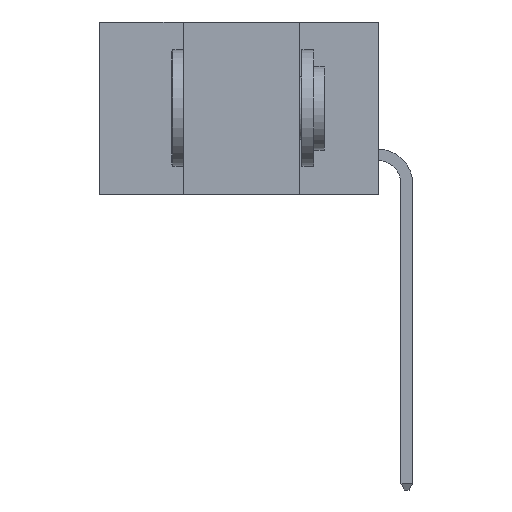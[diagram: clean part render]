
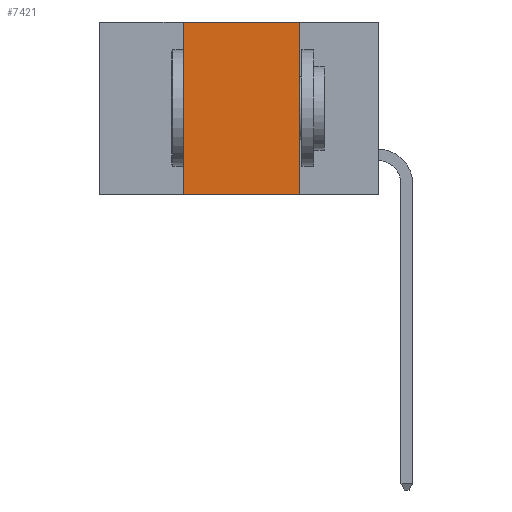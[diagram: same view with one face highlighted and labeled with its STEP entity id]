
A CAD part, left-side view. The second image highlights one B-rep face of the part: STEP entity #7421.
In plain terms, the highlighted planar face has unit normal (-1, 0, 0).
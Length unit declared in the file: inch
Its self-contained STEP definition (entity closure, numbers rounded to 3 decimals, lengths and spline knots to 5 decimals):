
#63 = LINE ( 'NONE', #23181, #14083 ) ;
#337 = CARTESIAN_POINT ( 'NONE',  ( 0., 0.17, -0.37 ) ) ;
#1043 = EDGE_CURVE ( 'NONE', #14700, #1186, #8381, .T. ) ;
#1186 = VERTEX_POINT ( 'NONE', #1383 ) ;
#1383 = CARTESIAN_POINT ( 'NONE',  ( 0., 0.17, -0.37 ) ) ;
#1869 = VECTOR ( 'NONE', #4277, 39.37008 ) ;
#3516 = EDGE_CURVE ( 'NONE', #14700, #6450, #6801, .T. ) ;
#4277 = DIRECTION ( 'NONE',  ( 0., 0., 1. ) ) ;
#4461 = DIRECTION ( 'NONE',  ( 0., 0., -1. ) ) ;
#6450 = VERTEX_POINT ( 'NONE', #11587 ) ;
#6664 = AXIS2_PLACEMENT_3D ( 'NONE', #16986, #16760, #16734 ) ;
#6705 = CARTESIAN_POINT ( 'NONE',  ( 0., 0.6, -0.37 ) ) ;
#6801 = LINE ( 'NONE', #8044, #1869 ) ;
#7071 = FACE_OUTER_BOUND ( 'NONE', #11452, .T. ) ;
#7185 = CARTESIAN_POINT ( 'NONE',  ( 0., 0.17, 0. ) ) ;
#7223 = VECTOR ( 'NONE', #11606, 39.37008 ) ;
#7421 = ADVANCED_FACE ( 'NONE', ( #7071 ), #16840, .F. ) ;
#8044 = CARTESIAN_POINT ( 'NONE',  ( 0., 0.42, -0.37 ) ) ;
#8247 = VERTEX_POINT ( 'NONE', #7185 ) ;
#8381 = LINE ( 'NONE', #6705, #7223 ) ;
#8441 = ORIENTED_EDGE ( 'NONE', *, *, #13353, .F. ) ;
#8505 = ORIENTED_EDGE ( 'NONE', *, *, #9731, .F. ) ;
#8618 = ORIENTED_EDGE ( 'NONE', *, *, #3516, .F. ) ;
#8644 = ORIENTED_EDGE ( 'NONE', *, *, #1043, .T. ) ;
#9731 = EDGE_CURVE ( 'NONE', #6450, #8247, #63, .T. ) ;
#11452 = EDGE_LOOP ( 'NONE', ( #8441, #8505, #8618, #8644 ) ) ;
#11587 = CARTESIAN_POINT ( 'NONE',  ( 0., 0.42, 0. ) ) ;
#11606 = DIRECTION ( 'NONE',  ( 0., -1., 0. ) ) ;
#13353 = EDGE_CURVE ( 'NONE', #8247, #1186, #18780, .T. ) ;
#14083 = VECTOR ( 'NONE', #21564, 39.37008 ) ;
#14700 = VERTEX_POINT ( 'NONE', #15480 ) ;
#15480 = CARTESIAN_POINT ( 'NONE',  ( 0., 0.42, -0.37 ) ) ;
#16734 = DIRECTION ( 'NONE',  ( 0., 0., -1. ) ) ;
#16760 = DIRECTION ( 'NONE',  ( 1., 0., 0. ) ) ;
#16840 = PLANE ( 'NONE',  #6664 ) ;
#16986 = CARTESIAN_POINT ( 'NONE',  ( 0., 0.6, 0. ) ) ;
#18780 = LINE ( 'NONE', #337, #22807 ) ;
#21564 = DIRECTION ( 'NONE',  ( 0., -1., 0. ) ) ;
#22807 = VECTOR ( 'NONE', #4461, 39.37008 ) ;
#23181 = CARTESIAN_POINT ( 'NONE',  ( 0., 0.6, 0. ) ) ;
